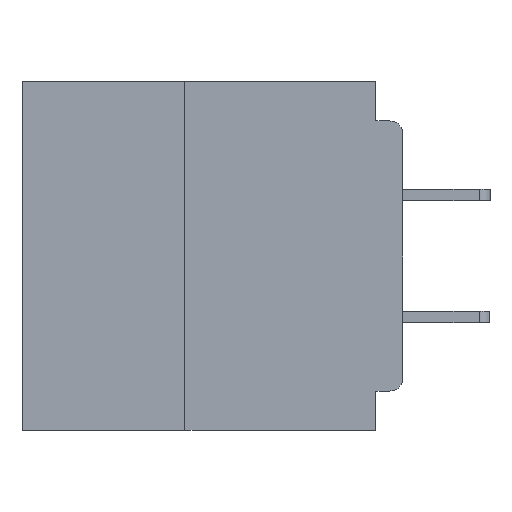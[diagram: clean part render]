
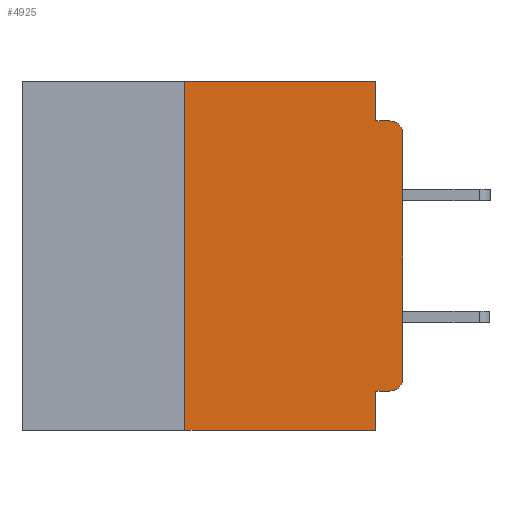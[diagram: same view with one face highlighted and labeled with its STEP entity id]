
A CAD part, left-side view. The second image highlights one B-rep face of the part: STEP entity #4925.
In plain terms, the highlighted planar face has unit normal (-1, 0, 0).
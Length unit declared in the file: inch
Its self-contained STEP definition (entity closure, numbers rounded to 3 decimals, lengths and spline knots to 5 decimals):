
#50 = FACE_OUTER_BOUND ( 'NONE', #24612, .T. ) ;
#99 = CARTESIAN_POINT ( 'NONE',  ( 0., 0.25, -0.4 ) ) ;
#313 = CARTESIAN_POINT ( 'NONE',  ( 0., 0.031, -0.4 ) ) ;
#902 = DIRECTION ( 'NONE',  ( 0., -1., 0. ) ) ;
#1146 = AXIS2_PLACEMENT_3D ( 'NONE', #9991, #17459, #43039 ) ;
#1616 = ORIENTED_EDGE ( 'NONE', *, *, #25208, .T. ) ;
#2329 = CARTESIAN_POINT ( 'NONE',  ( 0., 0., 0. ) ) ;
#2883 = CARTESIAN_POINT ( 'NONE',  ( 0., 0.437, 0. ) ) ;
#3832 = VERTEX_POINT ( 'NONE', #99 ) ;
#4185 = CARTESIAN_POINT ( 'NONE',  ( 0., 0.015, -0.34 ) ) ;
#4238 = CIRCLE ( 'NONE', #21279, 0.015 ) ;
#4925 = ADVANCED_FACE ( 'NONE', ( #50 ), #42727, .F. ) ;
#5363 = DIRECTION ( 'NONE',  ( 0., -1., 0. ) ) ;
#6087 = DIRECTION ( 'NONE',  ( 0., 0., 1. ) ) ;
#6229 = VECTOR ( 'NONE', #902, 39.37008 ) ;
#6538 = ORIENTED_EDGE ( 'NONE', *, *, #39831, .F. ) ;
#6645 = VERTEX_POINT ( 'NONE', #38921 ) ;
#6797 = CARTESIAN_POINT ( 'NONE',  ( 0., 0.015, -0.355 ) ) ;
#6986 = LINE ( 'NONE', #13384, #44907 ) ;
#7923 = DIRECTION ( 'NONE',  ( 0., 0., -1. ) ) ;
#8253 = VERTEX_POINT ( 'NONE', #14390 ) ;
#8328 = DIRECTION ( 'NONE',  ( -1., 0., 0. ) ) ;
#8380 = CIRCLE ( 'NONE', #16941, 0.015 ) ;
#9640 = ORIENTED_EDGE ( 'NONE', *, *, #42759, .F. ) ;
#9991 = CARTESIAN_POINT ( 'NONE',  ( 0., 0.437, 0. ) ) ;
#10139 = LINE ( 'NONE', #2883, #18883 ) ;
#12784 = EDGE_CURVE ( 'NONE', #29255, #14568, #18396, .T. ) ;
#12849 = VECTOR ( 'NONE', #40035, 39.37008 ) ;
#13384 = CARTESIAN_POINT ( 'NONE',  ( 0., 0.25, -0.4 ) ) ;
#14307 = LINE ( 'NONE', #2329, #32705 ) ;
#14390 = CARTESIAN_POINT ( 'NONE',  ( 0., 0.031, 0. ) ) ;
#14568 = VERTEX_POINT ( 'NONE', #18537 ) ;
#15099 = VECTOR ( 'NONE', #5363, 39.37008 ) ;
#15571 = ORIENTED_EDGE ( 'NONE', *, *, #47520, .T. ) ;
#16941 = AXIS2_PLACEMENT_3D ( 'NONE', #30436, #8328, #34084 ) ;
#17459 = DIRECTION ( 'NONE',  ( 1., 0., 0. ) ) ;
#18355 = CARTESIAN_POINT ( 'NONE',  ( 0., 0.015, -0.045 ) ) ;
#18396 = LINE ( 'NONE', #313, #27018 ) ;
#18537 = CARTESIAN_POINT ( 'NONE',  ( 0., 0.031, -0.4 ) ) ;
#18883 = VECTOR ( 'NONE', #32404, 39.37008 ) ;
#21279 = AXIS2_PLACEMENT_3D ( 'NONE', #4185, #30007, #7923 ) ;
#21421 = VERTEX_POINT ( 'NONE', #18355 ) ;
#22159 = EDGE_CURVE ( 'NONE', #42806, #34023, #4238, .T. ) ;
#22399 = LINE ( 'NONE', #33246, #40660 ) ;
#23313 = ORIENTED_EDGE ( 'NONE', *, *, #34733, .F. ) ;
#23838 = CARTESIAN_POINT ( 'NONE',  ( 0., 0., -0.045 ) ) ;
#23934 = ORIENTED_EDGE ( 'NONE', *, *, #42273, .F. ) ;
#24612 = EDGE_LOOP ( 'NONE', ( #39260, #15571, #23313, #23934, #9640, #6538, #1616, #28265, #33217, #30808 ) ) ;
#25208 = EDGE_CURVE ( 'NONE', #3832, #14568, #34444, .T. ) ;
#25406 = CARTESIAN_POINT ( 'NONE',  ( 0., 0., -0.355 ) ) ;
#25471 = EDGE_CURVE ( 'NONE', #34023, #41657, #14307, .T. ) ;
#25780 = CARTESIAN_POINT ( 'NONE',  ( 0., 0.25, 0. ) ) ;
#27018 = VECTOR ( 'NONE', #33593, 39.37008 ) ;
#28236 = DIRECTION ( 'NONE',  ( 0., 0., 1. ) ) ;
#28265 = ORIENTED_EDGE ( 'NONE', *, *, #12784, .F. ) ;
#29255 = VERTEX_POINT ( 'NONE', #36927 ) ;
#29661 = CARTESIAN_POINT ( 'NONE',  ( 0., 0., -0.06 ) ) ;
#30007 = DIRECTION ( 'NONE',  ( -1., 0., 0. ) ) ;
#30436 = CARTESIAN_POINT ( 'NONE',  ( 0., 0.015, -0.06 ) ) ;
#30808 = ORIENTED_EDGE ( 'NONE', *, *, #22159, .T. ) ;
#32404 = DIRECTION ( 'NONE',  ( 0., -1., 0. ) ) ;
#32705 = VECTOR ( 'NONE', #6087, 39.37008 ) ;
#33193 = EDGE_CURVE ( 'NONE', #42806, #29255, #44398, .T. ) ;
#33217 = ORIENTED_EDGE ( 'NONE', *, *, #33193, .F. ) ;
#33246 = CARTESIAN_POINT ( 'NONE',  ( 0., 0.031, 0. ) ) ;
#33593 = DIRECTION ( 'NONE',  ( 0., 0., -1. ) ) ;
#34023 = VERTEX_POINT ( 'NONE', #44932 ) ;
#34084 = DIRECTION ( 'NONE',  ( 0., 0., -1. ) ) ;
#34444 = LINE ( 'NONE', #37643, #6229 ) ;
#34733 = EDGE_CURVE ( 'NONE', #6645, #21421, #44311, .T. ) ;
#36905 = DIRECTION ( 'NONE',  ( 0., 0., -1. ) ) ;
#36927 = CARTESIAN_POINT ( 'NONE',  ( 0., 0.031, -0.355 ) ) ;
#37643 = CARTESIAN_POINT ( 'NONE',  ( 0., 0.437, -0.4 ) ) ;
#38921 = CARTESIAN_POINT ( 'NONE',  ( 0., 0.031, -0.045 ) ) ;
#39260 = ORIENTED_EDGE ( 'NONE', *, *, #25471, .T. ) ;
#39831 = EDGE_CURVE ( 'NONE', #3832, #42242, #6986, .T. ) ;
#40035 = DIRECTION ( 'NONE',  ( 0., 1., 0. ) ) ;
#40660 = VECTOR ( 'NONE', #36905, 39.37008 ) ;
#41657 = VERTEX_POINT ( 'NONE', #29661 ) ;
#42242 = VERTEX_POINT ( 'NONE', #25780 ) ;
#42273 = EDGE_CURVE ( 'NONE', #8253, #6645, #22399, .T. ) ;
#42727 = PLANE ( 'NONE',  #1146 ) ;
#42759 = EDGE_CURVE ( 'NONE', #42242, #8253, #10139, .T. ) ;
#42806 = VERTEX_POINT ( 'NONE', #6797 ) ;
#43039 = DIRECTION ( 'NONE',  ( 0., 0., -1. ) ) ;
#44311 = LINE ( 'NONE', #23838, #15099 ) ;
#44398 = LINE ( 'NONE', #25406, #12849 ) ;
#44907 = VECTOR ( 'NONE', #28236, 39.37008 ) ;
#44932 = CARTESIAN_POINT ( 'NONE',  ( 0., 0., -0.34 ) ) ;
#47520 = EDGE_CURVE ( 'NONE', #41657, #21421, #8380, .T. ) ;
